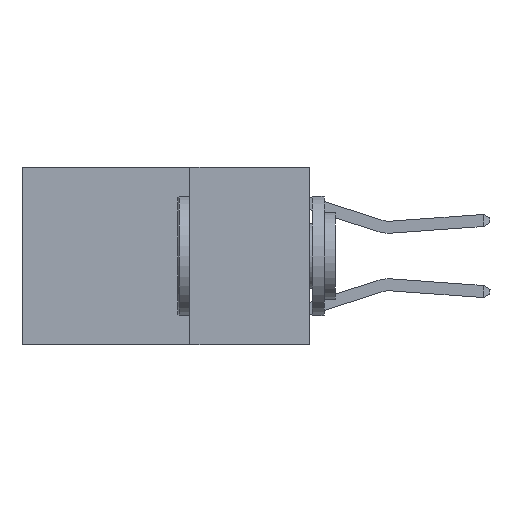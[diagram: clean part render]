
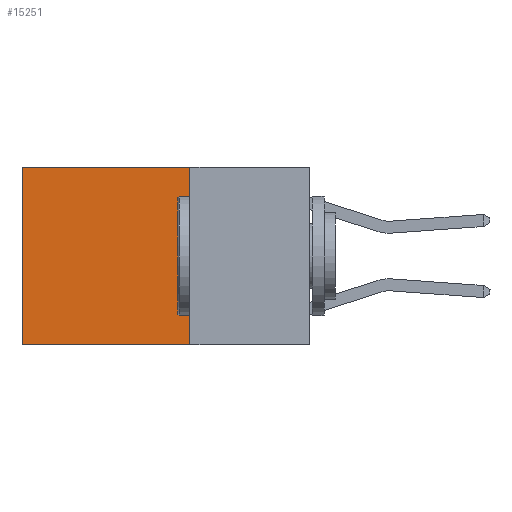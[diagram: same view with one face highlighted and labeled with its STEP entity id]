
A CAD part, left-side view. The second image highlights one B-rep face of the part: STEP entity #15251.
In plain terms, the highlighted planar face has unit normal (-1, 0, 0).
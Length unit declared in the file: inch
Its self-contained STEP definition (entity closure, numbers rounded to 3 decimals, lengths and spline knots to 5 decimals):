
#1271 = DIRECTION ( 'NONE',  ( 0., 0., -1. ) ) ;
#1539 = DIRECTION ( 'NONE',  ( 0., 0., -1. ) ) ;
#1794 = VECTOR ( 'NONE', #1271, 39.37008 ) ;
#2042 = VERTEX_POINT ( 'NONE', #12536 ) ;
#2332 = AXIS2_PLACEMENT_3D ( 'NONE', #8625, #4169, #5800 ) ;
#2878 = LINE ( 'NONE', #17481, #3799 ) ;
#3006 = DIRECTION ( 'NONE',  ( 0., 1., 0. ) ) ;
#3489 = LINE ( 'NONE', #15168, #1794 ) ;
#3772 = EDGE_CURVE ( 'NONE', #2042, #5146, #3489, .T. ) ;
#3799 = VECTOR ( 'NONE', #14554, 39.37008 ) ;
#3969 = EDGE_CURVE ( 'NONE', #4929, #5146, #2878, .T. ) ;
#4169 = DIRECTION ( 'NONE',  ( 1., 0., 0. ) ) ;
#4364 = CARTESIAN_POINT ( 'NONE',  ( 0.2625, 0.25, 0. ) ) ;
#4483 = LINE ( 'NONE', #8855, #16679 ) ;
#4845 = VERTEX_POINT ( 'NONE', #4364 ) ;
#4929 = VERTEX_POINT ( 'NONE', #5594 ) ;
#5146 = VERTEX_POINT ( 'NONE', #9669 ) ;
#5297 = EDGE_CURVE ( 'NONE', #4845, #2042, #8523, .T. ) ;
#5511 = PLANE ( 'NONE',  #2332 ) ;
#5594 = CARTESIAN_POINT ( 'NONE',  ( 0.2625, 0.25, -0.37 ) ) ;
#5800 = DIRECTION ( 'NONE',  ( 0., 0., -1. ) ) ;
#8523 = LINE ( 'NONE', #16001, #18019 ) ;
#8625 = CARTESIAN_POINT ( 'NONE',  ( 0.2625, 0.25, 0. ) ) ;
#8855 = CARTESIAN_POINT ( 'NONE',  ( 0.2625, 0.25, 0. ) ) ;
#9669 = CARTESIAN_POINT ( 'NONE',  ( 0.2625, 0.6, -0.37 ) ) ;
#9900 = ORIENTED_EDGE ( 'NONE', *, *, #14565, .F. ) ;
#10059 = ORIENTED_EDGE ( 'NONE', *, *, #3772, .T. ) ;
#11219 = FACE_OUTER_BOUND ( 'NONE', #12944, .T. ) ;
#12536 = CARTESIAN_POINT ( 'NONE',  ( 0.2625, 0.6, 0. ) ) ;
#12944 = EDGE_LOOP ( 'NONE', ( #10059, #15332, #9900, #15685 ) ) ;
#14554 = DIRECTION ( 'NONE',  ( 0., 1., 0. ) ) ;
#14565 = EDGE_CURVE ( 'NONE', #4845, #4929, #4483, .T. ) ;
#15168 = CARTESIAN_POINT ( 'NONE',  ( 0.2625, 0.6, 0. ) ) ;
#15251 = ADVANCED_FACE ( 'NONE', ( #11219 ), #5511, .F. ) ;
#15332 = ORIENTED_EDGE ( 'NONE', *, *, #3969, .F. ) ;
#15685 = ORIENTED_EDGE ( 'NONE', *, *, #5297, .T. ) ;
#16001 = CARTESIAN_POINT ( 'NONE',  ( 0.2625, 0.25, 0. ) ) ;
#16679 = VECTOR ( 'NONE', #1539, 39.37008 ) ;
#17481 = CARTESIAN_POINT ( 'NONE',  ( 0.2625, 0.25, -0.37 ) ) ;
#18019 = VECTOR ( 'NONE', #3006, 39.37008 ) ;
